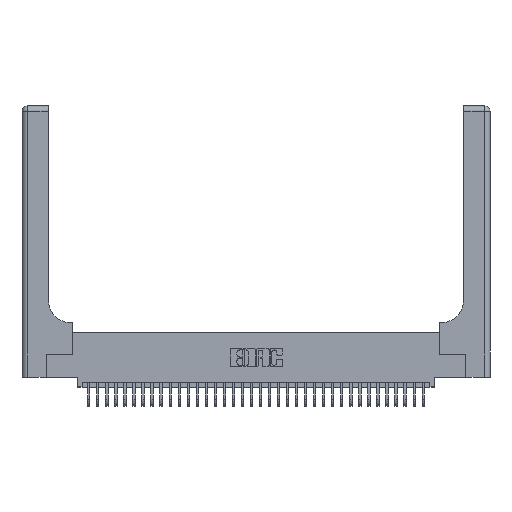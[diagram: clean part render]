
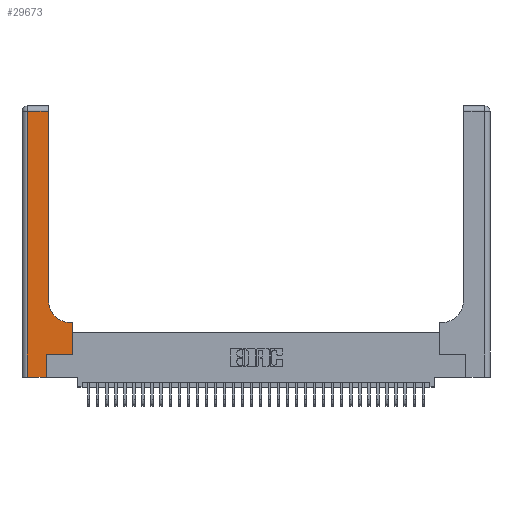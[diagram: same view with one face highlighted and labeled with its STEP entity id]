
A CAD part, top view. The second image highlights one B-rep face of the part: STEP entity #29673.
In plain terms, the highlighted planar face has unit normal (0, 0, 1).
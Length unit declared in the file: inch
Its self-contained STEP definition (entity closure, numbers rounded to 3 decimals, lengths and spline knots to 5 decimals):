
#669 = DIRECTION ( 'NONE',  ( -1., 0., 0. ) ) ;
#1171 = VECTOR ( 'NONE', #30075, 39.37008 ) ;
#2837 = CARTESIAN_POINT ( 'NONE',  ( 0.269, 0.25, 0.37 ) ) ;
#3010 = LINE ( 'NONE', #27221, #1171 ) ;
#3492 = PLANE ( 'NONE',  #32888 ) ;
#3613 = CARTESIAN_POINT ( 'NONE',  ( 0., 3., 0.37 ) ) ;
#3619 = ORIENTED_EDGE ( 'NONE', *, *, #26027, .T. ) ;
#3976 = EDGE_LOOP ( 'NONE', ( #29290, #20820, #27610, #3619, #16823, #28519, #10537, #15437, #13123 ) ) ;
#4467 = CARTESIAN_POINT ( 'NONE',  ( 0.269, 0.25, 0.37 ) ) ;
#4590 = DIRECTION ( 'NONE',  ( 1., 0., 0. ) ) ;
#4806 = CARTESIAN_POINT ( 'NONE',  ( 0.5585, 0.25, 0.37 ) ) ;
#6142 = CARTESIAN_POINT ( 'NONE',  ( 0.06, 2.94, 0.37 ) ) ;
#6491 = DIRECTION ( 'NONE',  ( 0., 0., -1. ) ) ;
#6798 = VECTOR ( 'NONE', #35206, 39.37008 ) ;
#7049 = VECTOR ( 'NONE', #36903, 39.37008 ) ;
#7102 = CARTESIAN_POINT ( 'NONE',  ( 0.2915, 3., 0.37 ) ) ;
#7135 = AXIS2_PLACEMENT_3D ( 'NONE', #9842, #30015, #12752 ) ;
#7534 = VERTEX_POINT ( 'NONE', #18484 ) ;
#9842 = CARTESIAN_POINT ( 'NONE',  ( 0.5415, 0.85, 0.37 ) ) ;
#10537 = ORIENTED_EDGE ( 'NONE', *, *, #33497, .T. ) ;
#10970 = VERTEX_POINT ( 'NONE', #2837 ) ;
#11292 = EDGE_CURVE ( 'NONE', #7534, #32651, #30813, .T. ) ;
#11327 = LINE ( 'NONE', #4467, #27622 ) ;
#12469 = CARTESIAN_POINT ( 'NONE',  ( 0.06, 3., 0.37 ) ) ;
#12752 = DIRECTION ( 'NONE',  ( 1., 0., 0. ) ) ;
#13123 = ORIENTED_EDGE ( 'NONE', *, *, #32407, .T. ) ;
#13295 = CARTESIAN_POINT ( 'NONE',  ( 0.06, 0., 0.37 ) ) ;
#13771 = CARTESIAN_POINT ( 'NONE',  ( 0.2915, 0.6, 0.37 ) ) ;
#14307 = LINE ( 'NONE', #13771, #27847 ) ;
#14530 = VECTOR ( 'NONE', #669, 39.37008 ) ;
#14535 = LINE ( 'NONE', #23770, #6798 ) ;
#15437 = ORIENTED_EDGE ( 'NONE', *, *, #24982, .T. ) ;
#15456 = LINE ( 'NONE', #23766, #14530 ) ;
#16724 = DIRECTION ( 'NONE',  ( -1., 0., 0. ) ) ;
#16823 = ORIENTED_EDGE ( 'NONE', *, *, #29157, .T. ) ;
#17132 = LINE ( 'NONE', #12469, #31460 ) ;
#18484 = CARTESIAN_POINT ( 'NONE',  ( 0.2915, 0.85, 0.37 ) ) ;
#19131 = CARTESIAN_POINT ( 'NONE',  ( 0.5415, 0.6, 0.37 ) ) ;
#20041 = VERTEX_POINT ( 'NONE', #4806 ) ;
#20820 = ORIENTED_EDGE ( 'NONE', *, *, #36722, .T. ) ;
#21346 = EDGE_CURVE ( 'NONE', #10970, #20041, #11327, .T. ) ;
#22511 = LINE ( 'NONE', #34031, #7049 ) ;
#23766 = CARTESIAN_POINT ( 'NONE',  ( 0., 2.94, 0.37 ) ) ;
#23770 = CARTESIAN_POINT ( 'NONE',  ( 0.269, 0., 0.37 ) ) ;
#24023 = DIRECTION ( 'NONE',  ( 0., -1., 0. ) ) ;
#24841 = CIRCLE ( 'NONE', #7135, 0.25 ) ;
#24982 = EDGE_CURVE ( 'NONE', #27357, #33863, #14307, .T. ) ;
#25653 = VERTEX_POINT ( 'NONE', #6142 ) ;
#26027 = EDGE_CURVE ( 'NONE', #26579, #30896, #22511, .T. ) ;
#26579 = VERTEX_POINT ( 'NONE', #13295 ) ;
#26750 = DIRECTION ( 'NONE',  ( -1., 0., 0. ) ) ;
#27221 = CARTESIAN_POINT ( 'NONE',  ( 0.5585, 0.25, 0.37 ) ) ;
#27357 = VERTEX_POINT ( 'NONE', #27886 ) ;
#27610 = ORIENTED_EDGE ( 'NONE', *, *, #31003, .T. ) ;
#27622 = VECTOR ( 'NONE', #4590, 39.37008 ) ;
#27847 = VECTOR ( 'NONE', #16724, 39.37008 ) ;
#27886 = CARTESIAN_POINT ( 'NONE',  ( 0.5585, 0.6, 0.37 ) ) ;
#28033 = FACE_OUTER_BOUND ( 'NONE', #3976, .T. ) ;
#28519 = ORIENTED_EDGE ( 'NONE', *, *, #21346, .T. ) ;
#29157 = EDGE_CURVE ( 'NONE', #30896, #10970, #14535, .T. ) ;
#29290 = ORIENTED_EDGE ( 'NONE', *, *, #11292, .T. ) ;
#29380 = CARTESIAN_POINT ( 'NONE',  ( 0.269, 0., 0.37 ) ) ;
#29673 = ADVANCED_FACE ( 'NONE', ( #28033 ), #3492, .F. ) ;
#30015 = DIRECTION ( 'NONE',  ( 0., 0., -1. ) ) ;
#30075 = DIRECTION ( 'NONE',  ( 0., 1., 0. ) ) ;
#30813 = LINE ( 'NONE', #7102, #31695 ) ;
#30896 = VERTEX_POINT ( 'NONE', #29380 ) ;
#31003 = EDGE_CURVE ( 'NONE', #25653, #26579, #17132, .T. ) ;
#31460 = VECTOR ( 'NONE', #24023, 39.37008 ) ;
#31695 = VECTOR ( 'NONE', #35772, 39.37008 ) ;
#32407 = EDGE_CURVE ( 'NONE', #33863, #7534, #24841, .T. ) ;
#32651 = VERTEX_POINT ( 'NONE', #36835 ) ;
#32888 = AXIS2_PLACEMENT_3D ( 'NONE', #3613, #6491, #26750 ) ;
#33497 = EDGE_CURVE ( 'NONE', #20041, #27357, #3010, .T. ) ;
#33863 = VERTEX_POINT ( 'NONE', #19131 ) ;
#34031 = CARTESIAN_POINT ( 'NONE',  ( 0., 0., 0.37 ) ) ;
#35206 = DIRECTION ( 'NONE',  ( 0., 1., 0. ) ) ;
#35772 = DIRECTION ( 'NONE',  ( 0., 1., 0. ) ) ;
#36722 = EDGE_CURVE ( 'NONE', #32651, #25653, #15456, .T. ) ;
#36835 = CARTESIAN_POINT ( 'NONE',  ( 0.2915, 2.94, 0.37 ) ) ;
#36903 = DIRECTION ( 'NONE',  ( 1., 0., 0. ) ) ;
